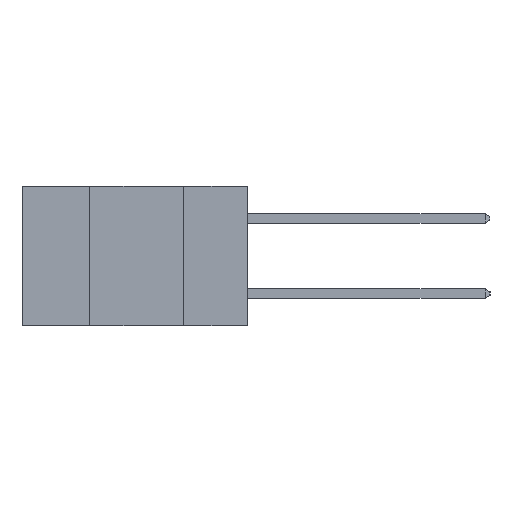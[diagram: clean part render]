
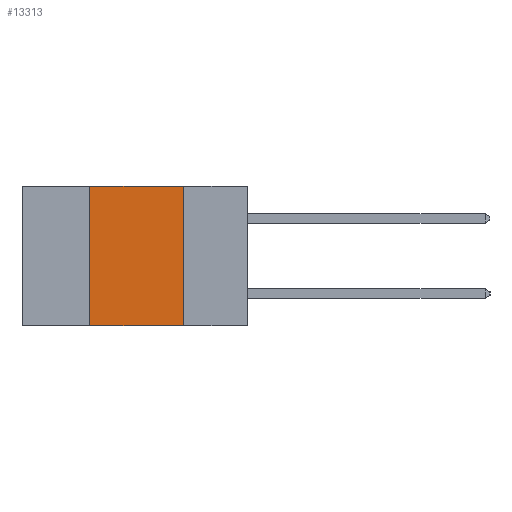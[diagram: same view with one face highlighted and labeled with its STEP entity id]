
A CAD part, left-side view. The second image highlights one B-rep face of the part: STEP entity #13313.
In plain terms, the highlighted planar face has unit normal (-1, 0, 0).
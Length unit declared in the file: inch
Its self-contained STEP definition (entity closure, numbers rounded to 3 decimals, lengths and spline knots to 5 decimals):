
#1377 = DIRECTION ( 'NONE',  ( 0., 0., -1. ) ) ;
#1834 = CARTESIAN_POINT ( 'NONE',  ( 0., 0.17, -0.37 ) ) ;
#1946 = PLANE ( 'NONE',  #12357 ) ;
#2289 = FACE_OUTER_BOUND ( 'NONE', #8970, .T. ) ;
#2435 = ORIENTED_EDGE ( 'NONE', *, *, #5082, .T. ) ;
#3306 = VECTOR ( 'NONE', #5783, 39.37008 ) ;
#3307 = EDGE_CURVE ( 'NONE', #8400, #9449, #6392, .T. ) ;
#3942 = VERTEX_POINT ( 'NONE', #10191 ) ;
#4254 = DIRECTION ( 'NONE',  ( 0., 0., -1. ) ) ;
#4397 = VECTOR ( 'NONE', #9579, 39.37008 ) ;
#4750 = ORIENTED_EDGE ( 'NONE', *, *, #12313, .F. ) ;
#4973 = VECTOR ( 'NONE', #10160, 39.37008 ) ;
#5082 = EDGE_CURVE ( 'NONE', #3942, #9449, #13256, .T. ) ;
#5144 = CARTESIAN_POINT ( 'NONE',  ( 0., 0.42, -0.37 ) ) ;
#5518 = CARTESIAN_POINT ( 'NONE',  ( 0., 0.42, 0. ) ) ;
#5761 = CARTESIAN_POINT ( 'NONE',  ( 0., 0.6, 0. ) ) ;
#5783 = DIRECTION ( 'NONE',  ( 0., 0., 1. ) ) ;
#6293 = LINE ( 'NONE', #5144, #3306 ) ;
#6392 = LINE ( 'NONE', #1834, #8972 ) ;
#6599 = EDGE_CURVE ( 'NONE', #3942, #12800, #6293, .T. ) ;
#7020 = ORIENTED_EDGE ( 'NONE', *, *, #3307, .F. ) ;
#7038 = CARTESIAN_POINT ( 'NONE',  ( 0., 0.17, 0. ) ) ;
#8400 = VERTEX_POINT ( 'NONE', #7038 ) ;
#8713 = CARTESIAN_POINT ( 'NONE',  ( 0., 0.17, -0.37 ) ) ;
#8970 = EDGE_LOOP ( 'NONE', ( #7020, #4750, #13250, #2435 ) ) ;
#8972 = VECTOR ( 'NONE', #1377, 39.37008 ) ;
#9449 = VERTEX_POINT ( 'NONE', #8713 ) ;
#9579 = DIRECTION ( 'NONE',  ( 0., -1., 0. ) ) ;
#9609 = CARTESIAN_POINT ( 'NONE',  ( 0., 0.6, -0.37 ) ) ;
#9771 = CARTESIAN_POINT ( 'NONE',  ( 0., 0.6, 0. ) ) ;
#10160 = DIRECTION ( 'NONE',  ( 0., -1., 0. ) ) ;
#10191 = CARTESIAN_POINT ( 'NONE',  ( 0., 0.42, -0.37 ) ) ;
#10803 = LINE ( 'NONE', #5761, #4973 ) ;
#10833 = DIRECTION ( 'NONE',  ( 1., 0., 0. ) ) ;
#12313 = EDGE_CURVE ( 'NONE', #12800, #8400, #10803, .T. ) ;
#12357 = AXIS2_PLACEMENT_3D ( 'NONE', #9771, #10833, #4254 ) ;
#12800 = VERTEX_POINT ( 'NONE', #5518 ) ;
#13250 = ORIENTED_EDGE ( 'NONE', *, *, #6599, .F. ) ;
#13256 = LINE ( 'NONE', #9609, #4397 ) ;
#13313 = ADVANCED_FACE ( 'NONE', ( #2289 ), #1946, .F. ) ;
